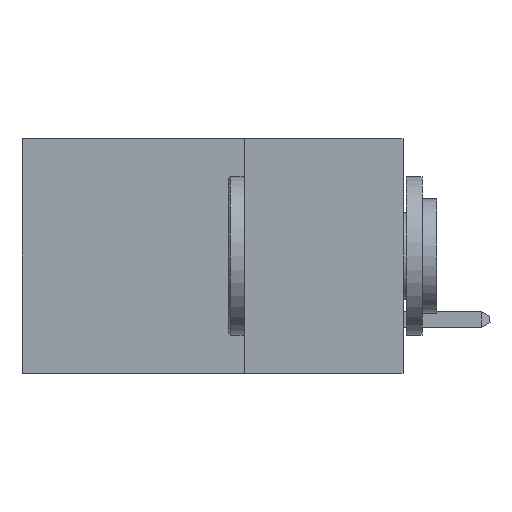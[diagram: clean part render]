
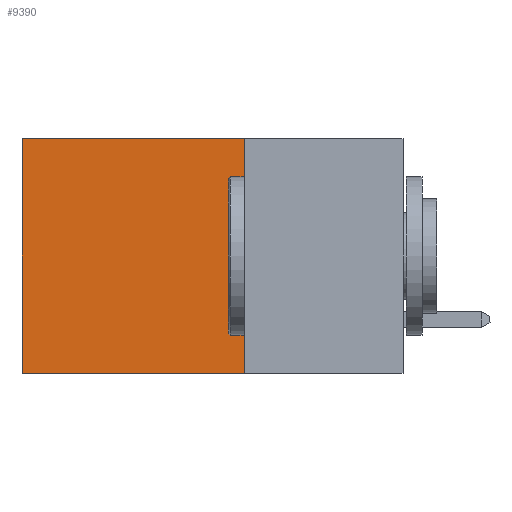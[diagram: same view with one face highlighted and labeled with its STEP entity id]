
A CAD part, left-side view. The second image highlights one B-rep face of the part: STEP entity #9390.
In plain terms, the highlighted planar face has unit normal (-1, 0, 0).
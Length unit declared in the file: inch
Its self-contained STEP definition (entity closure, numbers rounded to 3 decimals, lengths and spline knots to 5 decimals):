
#837 = CARTESIAN_POINT ( 'NONE',  ( 0.2875, 0.25, 0. ) ) ;
#874 = ORIENTED_EDGE ( 'NONE', *, *, #9720, .T. ) ;
#1862 = ORIENTED_EDGE ( 'NONE', *, *, #21215, .F. ) ;
#1940 = AXIS2_PLACEMENT_3D ( 'NONE', #837, #5194, #19529 ) ;
#2257 = EDGE_LOOP ( 'NONE', ( #874, #12188, #1862, #20459 ) ) ;
#3031 = PLANE ( 'NONE',  #1940 ) ;
#3196 = VERTEX_POINT ( 'NONE', #17970 ) ;
#4988 = EDGE_CURVE ( 'NONE', #5649, #21830, #13580, .T. ) ;
#5194 = DIRECTION ( 'NONE',  ( 1., 0., 0. ) ) ;
#5426 = CARTESIAN_POINT ( 'NONE',  ( 0.2875, 0.25, 0. ) ) ;
#5649 = VERTEX_POINT ( 'NONE', #24680 ) ;
#7941 = CARTESIAN_POINT ( 'NONE',  ( 0.2875, 0.25, -0.37 ) ) ;
#9390 = ADVANCED_FACE ( 'NONE', ( #17738 ), #3031, .F. ) ;
#9720 = EDGE_CURVE ( 'NONE', #21830, #11136, #26281, .T. ) ;
#10029 = DIRECTION ( 'NONE',  ( 0., 1., 0. ) ) ;
#11136 = VERTEX_POINT ( 'NONE', #19083 ) ;
#12188 = ORIENTED_EDGE ( 'NONE', *, *, #25464, .F. ) ;
#12513 = CARTESIAN_POINT ( 'NONE',  ( 0.2875, 0.25, 0. ) ) ;
#12621 = LINE ( 'NONE', #7941, #17943 ) ;
#13580 = LINE ( 'NONE', #5426, #16982 ) ;
#16419 = DIRECTION ( 'NONE',  ( 0., 0., -1. ) ) ;
#16453 = VECTOR ( 'NONE', #18647, 39.37008 ) ;
#16934 = CARTESIAN_POINT ( 'NONE',  ( 0.2875, 0.6, 0. ) ) ;
#16982 = VECTOR ( 'NONE', #19764, 39.37008 ) ;
#17738 = FACE_OUTER_BOUND ( 'NONE', #2257, .T. ) ;
#17943 = VECTOR ( 'NONE', #10029, 39.37008 ) ;
#17970 = CARTESIAN_POINT ( 'NONE',  ( 0.2875, 0.25, -0.37 ) ) ;
#18647 = DIRECTION ( 'NONE',  ( 0., 0., -1. ) ) ;
#19083 = CARTESIAN_POINT ( 'NONE',  ( 0.2875, 0.6, -0.37 ) ) ;
#19529 = DIRECTION ( 'NONE',  ( 0., 0., -1. ) ) ;
#19764 = DIRECTION ( 'NONE',  ( 0., 1., 0. ) ) ;
#20459 = ORIENTED_EDGE ( 'NONE', *, *, #4988, .T. ) ;
#21215 = EDGE_CURVE ( 'NONE', #5649, #3196, #21843, .T. ) ;
#21830 = VERTEX_POINT ( 'NONE', #16934 ) ;
#21843 = LINE ( 'NONE', #12513, #16453 ) ;
#22179 = VECTOR ( 'NONE', #16419, 39.37008 ) ;
#22459 = CARTESIAN_POINT ( 'NONE',  ( 0.2875, 0.6, 0. ) ) ;
#24680 = CARTESIAN_POINT ( 'NONE',  ( 0.2875, 0.25, 0. ) ) ;
#25464 = EDGE_CURVE ( 'NONE', #3196, #11136, #12621, .T. ) ;
#26281 = LINE ( 'NONE', #22459, #22179 ) ;
